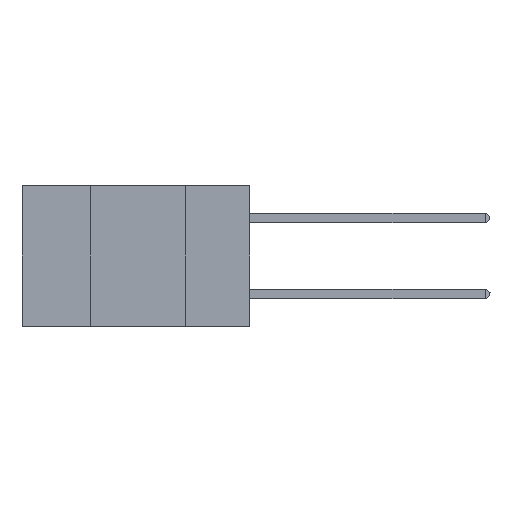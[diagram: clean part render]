
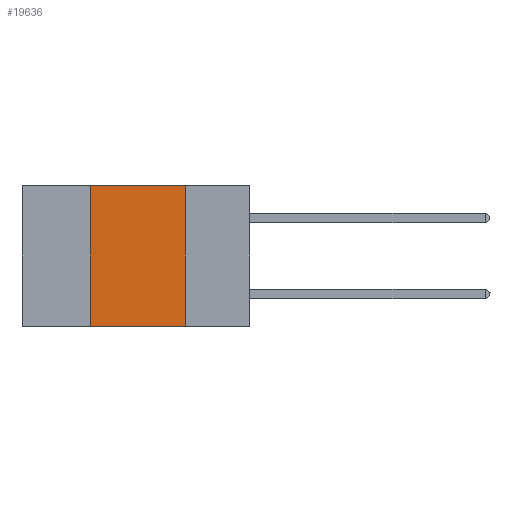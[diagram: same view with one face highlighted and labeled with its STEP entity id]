
A CAD part, left-side view. The second image highlights one B-rep face of the part: STEP entity #19636.
In plain terms, the highlighted planar face has unit normal (-1, 0, 0).
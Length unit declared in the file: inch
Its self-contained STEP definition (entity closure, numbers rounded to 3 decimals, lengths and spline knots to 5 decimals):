
#1083 = VECTOR ( 'NONE', #28678, 39.37008 ) ;
#3005 = CARTESIAN_POINT ( 'NONE',  ( 0., 0.6, 0. ) ) ;
#3714 = AXIS2_PLACEMENT_3D ( 'NONE', #16812, #25659, #25792 ) ;
#6804 = LINE ( 'NONE', #23702, #7729 ) ;
#7516 = VERTEX_POINT ( 'NONE', #22447 ) ;
#7729 = VECTOR ( 'NONE', #29469, 39.37008 ) ;
#7769 = CARTESIAN_POINT ( 'NONE',  ( 0., 0.42, 0. ) ) ;
#7946 = EDGE_LOOP ( 'NONE', ( #26501, #14325, #20704, #17883 ) ) ;
#9249 = LINE ( 'NONE', #21160, #27509 ) ;
#9698 = VERTEX_POINT ( 'NONE', #7769 ) ;
#10392 = FACE_OUTER_BOUND ( 'NONE', #7946, .T. ) ;
#10615 = LINE ( 'NONE', #3005, #1083 ) ;
#12322 = EDGE_CURVE ( 'NONE', #24523, #7516, #18579, .T. ) ;
#12934 = DIRECTION ( 'NONE',  ( 0., -1., 0. ) ) ;
#14325 = ORIENTED_EDGE ( 'NONE', *, *, #31161, .F. ) ;
#16812 = CARTESIAN_POINT ( 'NONE',  ( 0., 0.6, 0. ) ) ;
#17696 = VECTOR ( 'NONE', #12934, 39.37008 ) ;
#17883 = ORIENTED_EDGE ( 'NONE', *, *, #12322, .T. ) ;
#18003 = DIRECTION ( 'NONE',  ( 0., 0., -1. ) ) ;
#18579 = LINE ( 'NONE', #26255, #17696 ) ;
#19451 = PLANE ( 'NONE',  #3714 ) ;
#19636 = ADVANCED_FACE ( 'NONE', ( #10392 ), #19451, .F. ) ;
#20704 = ORIENTED_EDGE ( 'NONE', *, *, #36110, .F. ) ;
#21160 = CARTESIAN_POINT ( 'NONE',  ( 0., 0.17, 0. ) ) ;
#22447 = CARTESIAN_POINT ( 'NONE',  ( 0., 0.17, -0.37 ) ) ;
#23402 = EDGE_CURVE ( 'NONE', #25229, #7516, #9249, .T. ) ;
#23702 = CARTESIAN_POINT ( 'NONE',  ( 0., 0.42, 0. ) ) ;
#24523 = VERTEX_POINT ( 'NONE', #33336 ) ;
#25229 = VERTEX_POINT ( 'NONE', #29635 ) ;
#25659 = DIRECTION ( 'NONE',  ( 1., 0., 0. ) ) ;
#25792 = DIRECTION ( 'NONE',  ( 0., 0., -1. ) ) ;
#26255 = CARTESIAN_POINT ( 'NONE',  ( 0., 0.6, -0.37 ) ) ;
#26501 = ORIENTED_EDGE ( 'NONE', *, *, #23402, .F. ) ;
#27509 = VECTOR ( 'NONE', #18003, 39.37008 ) ;
#28678 = DIRECTION ( 'NONE',  ( 0., -1., 0. ) ) ;
#29469 = DIRECTION ( 'NONE',  ( 0., 0., 1. ) ) ;
#29635 = CARTESIAN_POINT ( 'NONE',  ( 0., 0.17, 0. ) ) ;
#31161 = EDGE_CURVE ( 'NONE', #9698, #25229, #10615, .T. ) ;
#33336 = CARTESIAN_POINT ( 'NONE',  ( 0., 0.42, -0.37 ) ) ;
#36110 = EDGE_CURVE ( 'NONE', #24523, #9698, #6804, .T. ) ;
